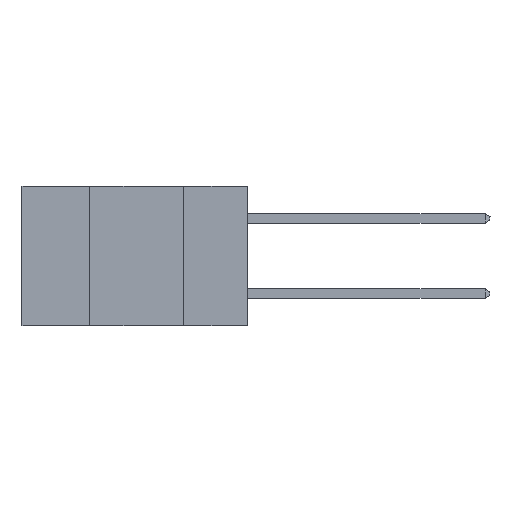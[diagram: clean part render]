
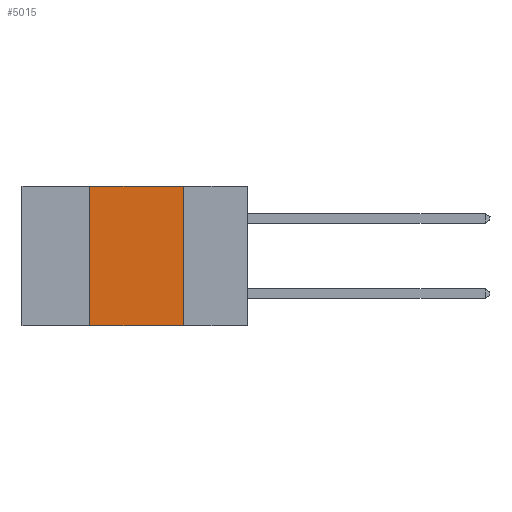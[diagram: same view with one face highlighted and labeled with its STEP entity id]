
A CAD part, left-side view. The second image highlights one B-rep face of the part: STEP entity #5015.
In plain terms, the highlighted planar face has unit normal (-1, 0, 0).
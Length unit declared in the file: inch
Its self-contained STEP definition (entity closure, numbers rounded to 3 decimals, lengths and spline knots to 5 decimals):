
#995 = VERTEX_POINT ( 'NONE', #15570 ) ;
#1264 = VECTOR ( 'NONE', #13224, 39.37008 ) ;
#1849 = CARTESIAN_POINT ( 'NONE',  ( 0., 0.17, 0. ) ) ;
#2831 = LINE ( 'NONE', #18942, #13175 ) ;
#2847 = EDGE_CURVE ( 'NONE', #995, #5878, #17782, .T. ) ;
#5015 = ADVANCED_FACE ( 'NONE', ( #11817 ), #14610, .F. ) ;
#5878 = VERTEX_POINT ( 'NONE', #1849 ) ;
#6273 = CARTESIAN_POINT ( 'NONE',  ( 0., 0.42, -0.37 ) ) ;
#6988 = CARTESIAN_POINT ( 'NONE',  ( 0., 0.6, -0.37 ) ) ;
#7473 = LINE ( 'NONE', #6988, #1264 ) ;
#7967 = EDGE_LOOP ( 'NONE', ( #20316, #16121, #9614, #22548 ) ) ;
#8178 = DIRECTION ( 'NONE',  ( 1., 0., 0. ) ) ;
#8184 = CARTESIAN_POINT ( 'NONE',  ( 0., 0.6, 0. ) ) ;
#8578 = DIRECTION ( 'NONE',  ( 0., 0., 1. ) ) ;
#8723 = CARTESIAN_POINT ( 'NONE',  ( 0., 0.17, -0.37 ) ) ;
#8888 = VECTOR ( 'NONE', #12103, 39.37008 ) ;
#9241 = DIRECTION ( 'NONE',  ( 0., 0., -1. ) ) ;
#9614 = ORIENTED_EDGE ( 'NONE', *, *, #15812, .F. ) ;
#9959 = CARTESIAN_POINT ( 'NONE',  ( 0., 0.6, 0. ) ) ;
#11638 = EDGE_CURVE ( 'NONE', #22986, #26753, #7473, .T. ) ;
#11817 = FACE_OUTER_BOUND ( 'NONE', #7967, .T. ) ;
#12103 = DIRECTION ( 'NONE',  ( 0., 0., -1. ) ) ;
#13175 = VECTOR ( 'NONE', #8578, 39.37008 ) ;
#13224 = DIRECTION ( 'NONE',  ( 0., -1., 0. ) ) ;
#14610 = PLANE ( 'NONE',  #21098 ) ;
#14911 = DIRECTION ( 'NONE',  ( 0., -1., 0. ) ) ;
#15570 = CARTESIAN_POINT ( 'NONE',  ( 0., 0.42, 0. ) ) ;
#15812 = EDGE_CURVE ( 'NONE', #22986, #995, #2831, .T. ) ;
#16121 = ORIENTED_EDGE ( 'NONE', *, *, #2847, .F. ) ;
#17782 = LINE ( 'NONE', #9959, #21920 ) ;
#18108 = EDGE_CURVE ( 'NONE', #5878, #26753, #19921, .T. ) ;
#18942 = CARTESIAN_POINT ( 'NONE',  ( 0., 0.42, 0. ) ) ;
#19921 = LINE ( 'NONE', #22404, #8888 ) ;
#20316 = ORIENTED_EDGE ( 'NONE', *, *, #18108, .F. ) ;
#21098 = AXIS2_PLACEMENT_3D ( 'NONE', #8184, #8178, #9241 ) ;
#21920 = VECTOR ( 'NONE', #14911, 39.37008 ) ;
#22404 = CARTESIAN_POINT ( 'NONE',  ( 0., 0.17, 0. ) ) ;
#22548 = ORIENTED_EDGE ( 'NONE', *, *, #11638, .T. ) ;
#22986 = VERTEX_POINT ( 'NONE', #6273 ) ;
#26753 = VERTEX_POINT ( 'NONE', #8723 ) ;
